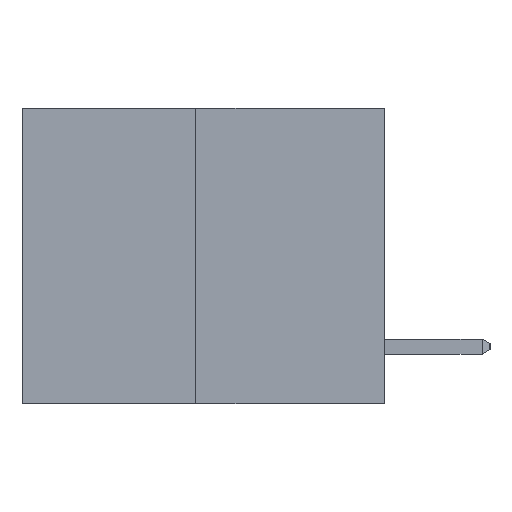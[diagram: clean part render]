
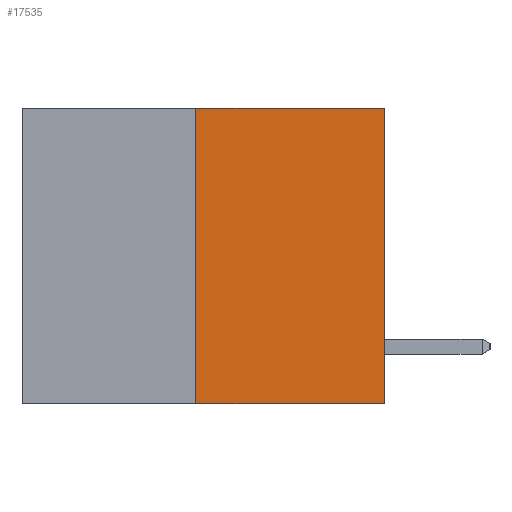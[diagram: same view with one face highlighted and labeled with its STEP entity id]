
A CAD part, left-side view. The second image highlights one B-rep face of the part: STEP entity #17535.
In plain terms, the highlighted planar face has unit normal (-1, 0, 0).
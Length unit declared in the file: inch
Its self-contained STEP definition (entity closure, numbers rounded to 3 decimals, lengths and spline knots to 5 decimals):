
#692 = EDGE_CURVE ( 'NONE', #24003, #22182, #11235, .T. ) ;
#910 = DIRECTION ( 'NONE',  ( 0., -1., 0. ) ) ;
#1127 = VECTOR ( 'NONE', #910, 39.37008 ) ;
#2790 = DIRECTION ( 'NONE',  ( 0., 0., -1. ) ) ;
#4109 = LINE ( 'NONE', #14655, #23604 ) ;
#5164 = CARTESIAN_POINT ( 'NONE',  ( 0., 0.6, -0.49 ) ) ;
#6407 = ORIENTED_EDGE ( 'NONE', *, *, #10202, .T. ) ;
#7415 = ORIENTED_EDGE ( 'NONE', *, *, #22099, .F. ) ;
#9368 = PLANE ( 'NONE',  #15919 ) ;
#10202 = EDGE_CURVE ( 'NONE', #13565, #22182, #23380, .T. ) ;
#10250 = VERTEX_POINT ( 'NONE', #21849 ) ;
#11146 = CARTESIAN_POINT ( 'NONE',  ( 0., 0., 0. ) ) ;
#11235 = LINE ( 'NONE', #16006, #26000 ) ;
#13118 = DIRECTION ( 'NONE',  ( 0., 0., 1. ) ) ;
#13565 = VERTEX_POINT ( 'NONE', #20214 ) ;
#13629 = EDGE_LOOP ( 'NONE', ( #7415, #25074, #6407, #13815 ) ) ;
#13815 = ORIENTED_EDGE ( 'NONE', *, *, #692, .F. ) ;
#14655 = CARTESIAN_POINT ( 'NONE',  ( 0., 0.312, -0.49 ) ) ;
#15721 = DIRECTION ( 'NONE',  ( 1., 0., 0. ) ) ;
#15919 = AXIS2_PLACEMENT_3D ( 'NONE', #24402, #15721, #2790 ) ;
#16006 = CARTESIAN_POINT ( 'NONE',  ( 0., 0.6, 0. ) ) ;
#17535 = ADVANCED_FACE ( 'NONE', ( #22081 ), #9368, .F. ) ;
#17744 = CARTESIAN_POINT ( 'NONE',  ( 0., 0., 0. ) ) ;
#17877 = DIRECTION ( 'NONE',  ( 0., -1., 0. ) ) ;
#18973 = DIRECTION ( 'NONE',  ( 0., 0., 1. ) ) ;
#20214 = CARTESIAN_POINT ( 'NONE',  ( 0., 0., -0.49 ) ) ;
#21107 = EDGE_CURVE ( 'NONE', #10250, #13565, #22997, .T. ) ;
#21849 = CARTESIAN_POINT ( 'NONE',  ( 0., 0.312, -0.49 ) ) ;
#22081 = FACE_OUTER_BOUND ( 'NONE', #13629, .T. ) ;
#22099 = EDGE_CURVE ( 'NONE', #10250, #24003, #4109, .T. ) ;
#22182 = VERTEX_POINT ( 'NONE', #17744 ) ;
#22997 = LINE ( 'NONE', #5164, #1127 ) ;
#23380 = LINE ( 'NONE', #11146, #23720 ) ;
#23604 = VECTOR ( 'NONE', #18973, 39.37008 ) ;
#23720 = VECTOR ( 'NONE', #13118, 39.37008 ) ;
#24003 = VERTEX_POINT ( 'NONE', #24056 ) ;
#24056 = CARTESIAN_POINT ( 'NONE',  ( 0., 0.312, 0. ) ) ;
#24402 = CARTESIAN_POINT ( 'NONE',  ( 0., 0.6, 0. ) ) ;
#25074 = ORIENTED_EDGE ( 'NONE', *, *, #21107, .T. ) ;
#26000 = VECTOR ( 'NONE', #17877, 39.37008 ) ;
